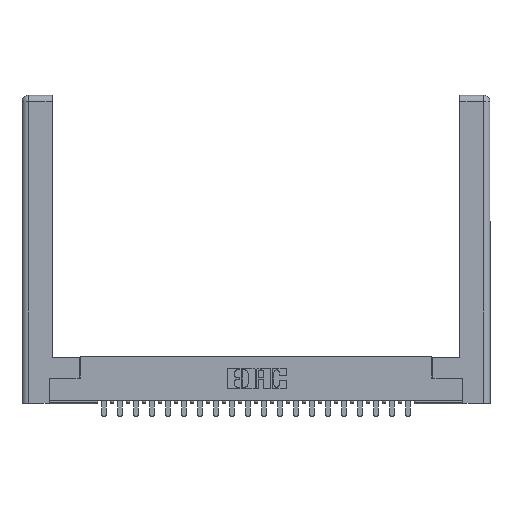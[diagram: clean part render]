
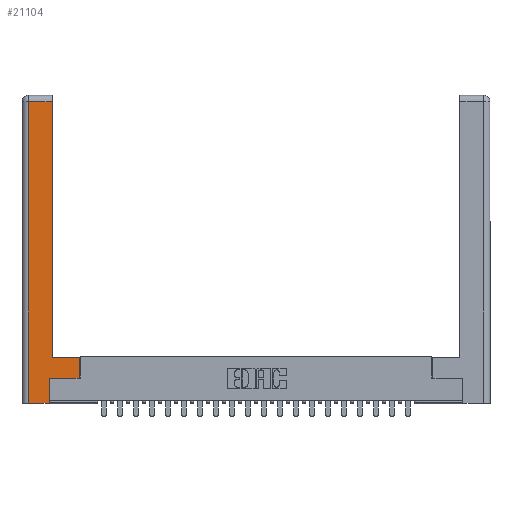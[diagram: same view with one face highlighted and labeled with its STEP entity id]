
A CAD part, top view. The second image highlights one B-rep face of the part: STEP entity #21104.
In plain terms, the highlighted planar face has unit normal (0, 0, 1).
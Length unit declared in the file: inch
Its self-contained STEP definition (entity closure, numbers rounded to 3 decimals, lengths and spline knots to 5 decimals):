
#483 = CARTESIAN_POINT ( 'NONE',  ( 0.0615, 0., 0. ) ) ;
#485 = LINE ( 'NONE', #483, #4380 ) ;
#571 = DIRECTION ( 'NONE',  ( 1., 0., 0. ) ) ;
#979 = DIRECTION ( 'NONE',  ( 0., -1., 0. ) ) ;
#1069 = VECTOR ( 'NONE', #19997, 39.37008 ) ;
#1398 = ORIENTED_EDGE ( 'NONE', *, *, #21667, .T. ) ;
#1430 = VECTOR ( 'NONE', #571, 39.37008 ) ;
#3043 = ORIENTED_EDGE ( 'NONE', *, *, #15312, .T. ) ;
#3104 = CARTESIAN_POINT ( 'NONE',  ( 0.565, 0.45, 0. ) ) ;
#3794 = EDGE_CURVE ( 'NONE', #8187, #13974, #26323, .T. ) ;
#4302 = LINE ( 'NONE', #25333, #14354 ) ;
#4380 = VECTOR ( 'NONE', #979, 39.37008 ) ;
#4645 = VERTEX_POINT ( 'NONE', #5033 ) ;
#5008 = CARTESIAN_POINT ( 'NONE',  ( 0., 0., 0. ) ) ;
#5033 = CARTESIAN_POINT ( 'NONE',  ( 0.565, 0.245, 0. ) ) ;
#5534 = CARTESIAN_POINT ( 'NONE',  ( 0.0615, 0., 0. ) ) ;
#5634 = CARTESIAN_POINT ( 'NONE',  ( 0.295, 3., 0. ) ) ;
#7944 = CARTESIAN_POINT ( 'NONE',  ( 0.295, 0.45, 0. ) ) ;
#8045 = ORIENTED_EDGE ( 'NONE', *, *, #15954, .T. ) ;
#8187 = VERTEX_POINT ( 'NONE', #5534 ) ;
#8371 = DIRECTION ( 'NONE',  ( 0., 1., 0. ) ) ;
#8535 = DIRECTION ( 'NONE',  ( 0., 1., 0. ) ) ;
#8556 = VERTEX_POINT ( 'NONE', #16182 ) ;
#8637 = ORIENTED_EDGE ( 'NONE', *, *, #23579, .T. ) ;
#8822 = CARTESIAN_POINT ( 'NONE',  ( 0.565, 0.245, 0. ) ) ;
#9358 = PLANE ( 'NONE',  #22759 ) ;
#10206 = DIRECTION ( 'NONE',  ( -1., 0., 0. ) ) ;
#11052 = CARTESIAN_POINT ( 'NONE',  ( 0.295, 0.45, 0. ) ) ;
#11608 = CARTESIAN_POINT ( 'NONE',  ( 0.0615, 2.94, 0. ) ) ;
#11674 = ORIENTED_EDGE ( 'NONE', *, *, #3794, .T. ) ;
#12067 = CARTESIAN_POINT ( 'NONE',  ( 0.265, 0., 0. ) ) ;
#13258 = VECTOR ( 'NONE', #8371, 39.37008 ) ;
#13260 = DIRECTION ( 'NONE',  ( 0., 0., -1. ) ) ;
#13422 = LINE ( 'NONE', #8822, #1430 ) ;
#13893 = LINE ( 'NONE', #18501, #13258 ) ;
#13974 = VERTEX_POINT ( 'NONE', #15883 ) ;
#14354 = VECTOR ( 'NONE', #8535, 39.37008 ) ;
#14596 = EDGE_CURVE ( 'NONE', #8556, #25062, #21871, .T. ) ;
#15312 = EDGE_CURVE ( 'NONE', #25182, #4645, #13422, .T. ) ;
#15406 = VECTOR ( 'NONE', #17760, 39.37008 ) ;
#15680 = ORIENTED_EDGE ( 'NONE', *, *, #17850, .T. ) ;
#15883 = CARTESIAN_POINT ( 'NONE',  ( 0.265, 0., 0. ) ) ;
#15954 = EDGE_CURVE ( 'NONE', #4645, #21168, #13893, .T. ) ;
#16182 = CARTESIAN_POINT ( 'NONE',  ( 0.295, 2.94, 0. ) ) ;
#16242 = DIRECTION ( 'NONE',  ( 0., 1., 0. ) ) ;
#17134 = VECTOR ( 'NONE', #10206, 39.37008 ) ;
#17760 = DIRECTION ( 'NONE',  ( -1., 0., 0. ) ) ;
#17850 = EDGE_CURVE ( 'NONE', #25062, #8187, #485, .T. ) ;
#18501 = CARTESIAN_POINT ( 'NONE',  ( 0.565, 0.45, 0. ) ) ;
#18787 = CARTESIAN_POINT ( 'NONE',  ( 0.265, 0.245, 0. ) ) ;
#19997 = DIRECTION ( 'NONE',  ( 1., 0., 0. ) ) ;
#20070 = CARTESIAN_POINT ( 'NONE',  ( 0.0615, 2.94, 0. ) ) ;
#20456 = ORIENTED_EDGE ( 'NONE', *, *, #14596, .T. ) ;
#20818 = LINE ( 'NONE', #5634, #26633 ) ;
#21104 = ADVANCED_FACE ( 'NONE', ( #23332 ), #9358, .F. ) ;
#21168 = VERTEX_POINT ( 'NONE', #3104 ) ;
#21337 = LINE ( 'NONE', #7944, #17134 ) ;
#21386 = DIRECTION ( 'NONE',  ( -1., 0., 0. ) ) ;
#21667 = EDGE_CURVE ( 'NONE', #21168, #24817, #21337, .T. ) ;
#21871 = LINE ( 'NONE', #11608, #15406 ) ;
#22759 = AXIS2_PLACEMENT_3D ( 'NONE', #5008, #13260, #21386 ) ;
#23270 = EDGE_CURVE ( 'NONE', #24817, #8556, #20818, .T. ) ;
#23332 = FACE_OUTER_BOUND ( 'NONE', #25622, .T. ) ;
#23579 = EDGE_CURVE ( 'NONE', #13974, #25182, #4302, .T. ) ;
#24612 = ORIENTED_EDGE ( 'NONE', *, *, #23270, .T. ) ;
#24817 = VERTEX_POINT ( 'NONE', #11052 ) ;
#25062 = VERTEX_POINT ( 'NONE', #20070 ) ;
#25182 = VERTEX_POINT ( 'NONE', #18787 ) ;
#25333 = CARTESIAN_POINT ( 'NONE',  ( 0.265, 0.245, 0. ) ) ;
#25622 = EDGE_LOOP ( 'NONE', ( #24612, #20456, #15680, #11674, #8637, #3043, #8045, #1398 ) ) ;
#26323 = LINE ( 'NONE', #12067, #1069 ) ;
#26633 = VECTOR ( 'NONE', #16242, 39.37008 ) ;
